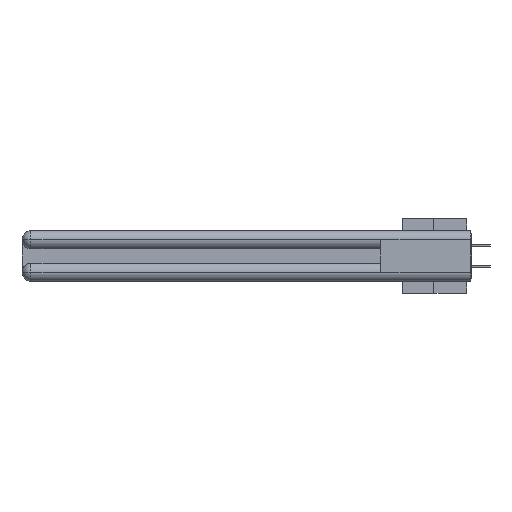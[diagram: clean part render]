
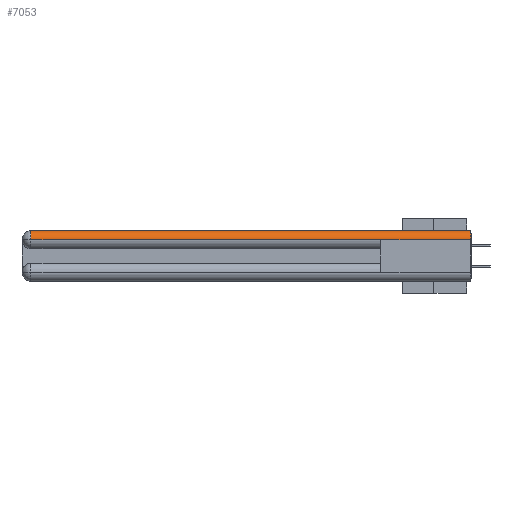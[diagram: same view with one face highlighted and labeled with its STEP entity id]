
A CAD part, left-side view. The second image highlights one B-rep face of the part: STEP entity #7053.
In plain terms, the highlighted cylindrical face has radius 1.562 mm (diameter 3.124 mm), a partial arc.
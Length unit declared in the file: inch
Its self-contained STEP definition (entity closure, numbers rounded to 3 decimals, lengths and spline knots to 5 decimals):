
#481 = CARTESIAN_POINT ( 'NONE',  ( 0., 2.94, -0.0615 ) ) ;
#532 = CARTESIAN_POINT ( 'NONE',  ( 0.0615, 0., 0. ) ) ;
#1906 = CARTESIAN_POINT ( 'NONE',  ( 0.0615, 0., -0.0615 ) ) ;
#2015 = DIRECTION ( 'NONE',  ( 1., 0., 0. ) ) ;
#2273 = CARTESIAN_POINT ( 'NONE',  ( 0., 3., -0.0615 ) ) ;
#3187 = CIRCLE ( 'NONE', #24710, 0.0615 ) ;
#3850 = ORIENTED_EDGE ( 'NONE', *, *, #13141, .T. ) ;
#4132 = CARTESIAN_POINT ( 'NONE',  ( 0.0615, 2.94, -0.0615 ) ) ;
#5027 = CIRCLE ( 'NONE', #5212, 0.0615 ) ;
#5212 = AXIS2_PLACEMENT_3D ( 'NONE', #1906, #29449, #2015 ) ;
#6456 = VERTEX_POINT ( 'NONE', #481 ) ;
#6855 = VERTEX_POINT ( 'NONE', #21558 ) ;
#7053 = ADVANCED_FACE ( 'NONE', ( #12579 ), #19883, .T. ) ;
#9666 = CARTESIAN_POINT ( 'NONE',  ( 0., 0., -0.0615 ) ) ;
#11390 = CARTESIAN_POINT ( 'NONE',  ( 0., 0.6, -0.0615 ) ) ;
#11421 = DIRECTION ( 'NONE',  ( 0., -1., 0. ) ) ;
#12174 = CARTESIAN_POINT ( 'NONE',  ( 0.0615, 2.94, 0. ) ) ;
#12432 = EDGE_CURVE ( 'NONE', #22427, #6456, #3187, .T. ) ;
#12579 = FACE_OUTER_BOUND ( 'NONE', #27954, .T. ) ;
#12912 = DIRECTION ( 'NONE',  ( 0., 1., 0. ) ) ;
#13141 = EDGE_CURVE ( 'NONE', #6456, #30610, #13688, .T. ) ;
#13421 = LINE ( 'NONE', #2273, #34843 ) ;
#13688 = LINE ( 'NONE', #34912, #28270 ) ;
#14274 = EDGE_CURVE ( 'NONE', #6855, #18563, #5027, .T. ) ;
#14569 = ORIENTED_EDGE ( 'NONE', *, *, #12432, .T. ) ;
#16635 = ORIENTED_EDGE ( 'NONE', *, *, #27176, .F. ) ;
#17913 = DIRECTION ( 'NONE',  ( 0., 0., 1. ) ) ;
#18058 = AXIS2_PLACEMENT_3D ( 'NONE', #32667, #32796, #27613 ) ;
#18563 = VERTEX_POINT ( 'NONE', #9666 ) ;
#19883 = CYLINDRICAL_SURFACE ( 'NONE', #18058, 0.0615 ) ;
#20052 = VECTOR ( 'NONE', #11421, 39.37008 ) ;
#20679 = DIRECTION ( 'NONE',  ( 0., -1., 0. ) ) ;
#21019 = ORIENTED_EDGE ( 'NONE', *, *, #24645, .F. ) ;
#21558 = CARTESIAN_POINT ( 'NONE',  ( 0.0615, 0., 0. ) ) ;
#22214 = LINE ( 'NONE', #532, #20052 ) ;
#22427 = VERTEX_POINT ( 'NONE', #12174 ) ;
#24645 = EDGE_CURVE ( 'NONE', #22427, #6855, #22214, .T. ) ;
#24710 = AXIS2_PLACEMENT_3D ( 'NONE', #4132, #20679, #17913 ) ;
#27176 = EDGE_CURVE ( 'NONE', #18563, #30610, #13421, .T. ) ;
#27311 = ORIENTED_EDGE ( 'NONE', *, *, #14274, .F. ) ;
#27613 = DIRECTION ( 'NONE',  ( 0., 0., 1. ) ) ;
#27954 = EDGE_LOOP ( 'NONE', ( #21019, #14569, #3850, #16635, #27311 ) ) ;
#28270 = VECTOR ( 'NONE', #29295, 39.37008 ) ;
#29295 = DIRECTION ( 'NONE',  ( 0., -1., 0. ) ) ;
#29449 = DIRECTION ( 'NONE',  ( 0., -1., 0. ) ) ;
#30610 = VERTEX_POINT ( 'NONE', #11390 ) ;
#32667 = CARTESIAN_POINT ( 'NONE',  ( 0.0615, 0., -0.0615 ) ) ;
#32796 = DIRECTION ( 'NONE',  ( 0., 1., 0. ) ) ;
#34843 = VECTOR ( 'NONE', #12912, 39.37008 ) ;
#34912 = CARTESIAN_POINT ( 'NONE',  ( 0., 3., -0.0615 ) ) ;
